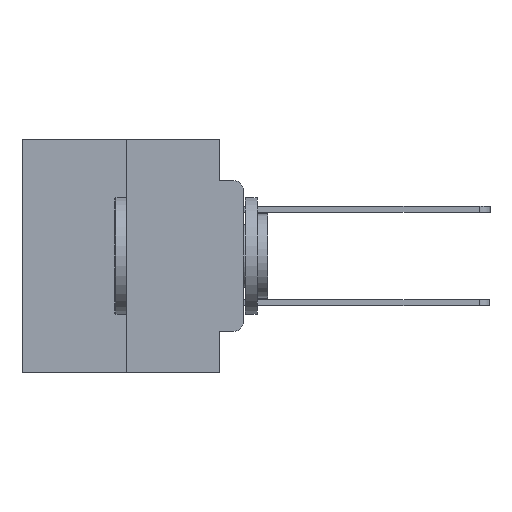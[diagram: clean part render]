
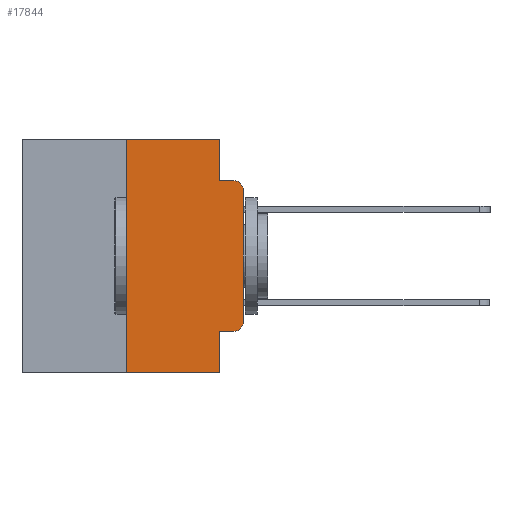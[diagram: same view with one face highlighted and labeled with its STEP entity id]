
A CAD part, left-side view. The second image highlights one B-rep face of the part: STEP entity #17844.
In plain terms, the highlighted planar face has unit normal (-1, 0, 0).
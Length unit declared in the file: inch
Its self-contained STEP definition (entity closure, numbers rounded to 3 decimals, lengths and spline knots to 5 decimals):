
#13 = EDGE_CURVE ( 'NONE', #25294, #18222, #15005, .T. ) ;
#178 = ORIENTED_EDGE ( 'NONE', *, *, #10089, .T. ) ;
#188 = CARTESIAN_POINT ( 'NONE',  ( 0., 0.051, 0. ) ) ;
#1223 = AXIS2_PLACEMENT_3D ( 'NONE', #18614, #5458, #20835 ) ;
#2082 = PLANE ( 'NONE',  #2248 ) ;
#2178 = VECTOR ( 'NONE', #22775, 39.37008 ) ;
#2248 = AXIS2_PLACEMENT_3D ( 'NONE', #13002, #26176, #4278 ) ;
#2723 = EDGE_CURVE ( 'NONE', #18222, #9395, #10074, .T. ) ;
#2893 = EDGE_CURVE ( 'NONE', #12361, #27998, #16249, .T. ) ;
#4278 = DIRECTION ( 'NONE',  ( 0., 0., -1. ) ) ;
#4590 = ORIENTED_EDGE ( 'NONE', *, *, #2893, .F. ) ;
#5425 = EDGE_CURVE ( 'NONE', #13084, #26789, #21064, .T. ) ;
#5458 = DIRECTION ( 'NONE',  ( -1., 0., 0. ) ) ;
#5539 = DIRECTION ( 'NONE',  ( 0., -1., 0. ) ) ;
#5814 = CARTESIAN_POINT ( 'NONE',  ( 0., 0.02, -0.0885 ) ) ;
#6116 = LINE ( 'NONE', #26170, #22265 ) ;
#6370 = DIRECTION ( 'NONE',  ( 0., 0., -1. ) ) ;
#6605 = VECTOR ( 'NONE', #15616, 39.37008 ) ;
#8033 = ORIENTED_EDGE ( 'NONE', *, *, #12316, .F. ) ;
#8049 = EDGE_CURVE ( 'NONE', #10988, #21113, #6116, .T. ) ;
#9182 = VECTOR ( 'NONE', #12582, 39.37008 ) ;
#9395 = VERTEX_POINT ( 'NONE', #26722 ) ;
#9638 = CARTESIAN_POINT ( 'NONE',  ( 0., 0., -0.1085 ) ) ;
#10074 = LINE ( 'NONE', #18649, #26225 ) ;
#10089 = EDGE_CURVE ( 'NONE', #26789, #27998, #11195, .T. ) ;
#10209 = DIRECTION ( 'NONE',  ( -1., 0., 0. ) ) ;
#10988 = VERTEX_POINT ( 'NONE', #25884 ) ;
#11195 = CIRCLE ( 'NONE', #1223, 0.02 ) ;
#11746 = CARTESIAN_POINT ( 'NONE',  ( 0., 0., -0.3915 ) ) ;
#11895 = CARTESIAN_POINT ( 'NONE',  ( 0., 0.473, -0.5 ) ) ;
#12191 = VECTOR ( 'NONE', #5539, 39.37008 ) ;
#12316 = EDGE_CURVE ( 'NONE', #9395, #12361, #24133, .T. ) ;
#12361 = VERTEX_POINT ( 'NONE', #22430 ) ;
#12582 = DIRECTION ( 'NONE',  ( 0., 0., 1. ) ) ;
#12856 = DIRECTION ( 'NONE',  ( 0., -1., 0. ) ) ;
#13002 = CARTESIAN_POINT ( 'NONE',  ( 0., 0.473, 0. ) ) ;
#13084 = VERTEX_POINT ( 'NONE', #11746 ) ;
#13384 = DIRECTION ( 'NONE',  ( 0., -1., 0. ) ) ;
#14019 = CARTESIAN_POINT ( 'NONE',  ( 0., 0.25, 0. ) ) ;
#14096 = DIRECTION ( 'NONE',  ( 0., -1., 0. ) ) ;
#14871 = LINE ( 'NONE', #11895, #25901 ) ;
#15005 = LINE ( 'NONE', #26072, #9182 ) ;
#15602 = ORIENTED_EDGE ( 'NONE', *, *, #25583, .T. ) ;
#15616 = DIRECTION ( 'NONE',  ( 0., 0., -1. ) ) ;
#16249 = LINE ( 'NONE', #19685, #22072 ) ;
#16430 = EDGE_CURVE ( 'NONE', #20726, #13084, #19118, .T. ) ;
#16604 = ORIENTED_EDGE ( 'NONE', *, *, #5425, .T. ) ;
#17455 = EDGE_LOOP ( 'NONE', ( #16604, #178, #4590, #8033, #25240, #25591, #15602, #25963, #18062, #22894 ) ) ;
#17585 = EDGE_CURVE ( 'NONE', #10988, #20726, #23183, .T. ) ;
#17844 = ADVANCED_FACE ( 'NONE', ( #27318 ), #2082, .F. ) ;
#18062 = ORIENTED_EDGE ( 'NONE', *, *, #17585, .T. ) ;
#18222 = VERTEX_POINT ( 'NONE', #14019 ) ;
#18614 = CARTESIAN_POINT ( 'NONE',  ( 0., 0.02, -0.1085 ) ) ;
#18649 = CARTESIAN_POINT ( 'NONE',  ( 0., 0.473, 0. ) ) ;
#19118 = CIRCLE ( 'NONE', #25589, 0.02 ) ;
#19685 = CARTESIAN_POINT ( 'NONE',  ( 0., 0.051, -0.0885 ) ) ;
#20726 = VERTEX_POINT ( 'NONE', #22937 ) ;
#20835 = DIRECTION ( 'NONE',  ( 0., 0., -1. ) ) ;
#21064 = LINE ( 'NONE', #21974, #2178 ) ;
#21113 = VERTEX_POINT ( 'NONE', #23858 ) ;
#21974 = CARTESIAN_POINT ( 'NONE',  ( 0., 0., 0. ) ) ;
#22072 = VECTOR ( 'NONE', #12856, 39.37008 ) ;
#22265 = VECTOR ( 'NONE', #6370, 39.37008 ) ;
#22430 = CARTESIAN_POINT ( 'NONE',  ( 0., 0.051, -0.0885 ) ) ;
#22775 = DIRECTION ( 'NONE',  ( 0., 0., 1. ) ) ;
#22894 = ORIENTED_EDGE ( 'NONE', *, *, #16430, .T. ) ;
#22937 = CARTESIAN_POINT ( 'NONE',  ( 0., 0.02, -0.4115 ) ) ;
#23183 = LINE ( 'NONE', #25339, #12191 ) ;
#23347 = CARTESIAN_POINT ( 'NONE',  ( 0., 0.02, -0.3915 ) ) ;
#23858 = CARTESIAN_POINT ( 'NONE',  ( 0., 0.051, -0.5 ) ) ;
#24002 = CARTESIAN_POINT ( 'NONE',  ( 0., 0.25, -0.5 ) ) ;
#24133 = LINE ( 'NONE', #188, #6605 ) ;
#25240 = ORIENTED_EDGE ( 'NONE', *, *, #2723, .F. ) ;
#25294 = VERTEX_POINT ( 'NONE', #24002 ) ;
#25339 = CARTESIAN_POINT ( 'NONE',  ( 0., 0.051, -0.4115 ) ) ;
#25574 = DIRECTION ( 'NONE',  ( 0., 0., -1. ) ) ;
#25583 = EDGE_CURVE ( 'NONE', #25294, #21113, #14871, .T. ) ;
#25589 = AXIS2_PLACEMENT_3D ( 'NONE', #23347, #10209, #25574 ) ;
#25591 = ORIENTED_EDGE ( 'NONE', *, *, #13, .F. ) ;
#25884 = CARTESIAN_POINT ( 'NONE',  ( 0., 0.051, -0.4115 ) ) ;
#25901 = VECTOR ( 'NONE', #14096, 39.37008 ) ;
#25963 = ORIENTED_EDGE ( 'NONE', *, *, #8049, .F. ) ;
#26072 = CARTESIAN_POINT ( 'NONE',  ( 0., 0.25, 0. ) ) ;
#26170 = CARTESIAN_POINT ( 'NONE',  ( 0., 0.051, 0. ) ) ;
#26176 = DIRECTION ( 'NONE',  ( 1., 0., 0. ) ) ;
#26225 = VECTOR ( 'NONE', #13384, 39.37008 ) ;
#26722 = CARTESIAN_POINT ( 'NONE',  ( 0., 0.051, 0. ) ) ;
#26789 = VERTEX_POINT ( 'NONE', #9638 ) ;
#27318 = FACE_OUTER_BOUND ( 'NONE', #17455, .T. ) ;
#27998 = VERTEX_POINT ( 'NONE', #5814 ) ;
